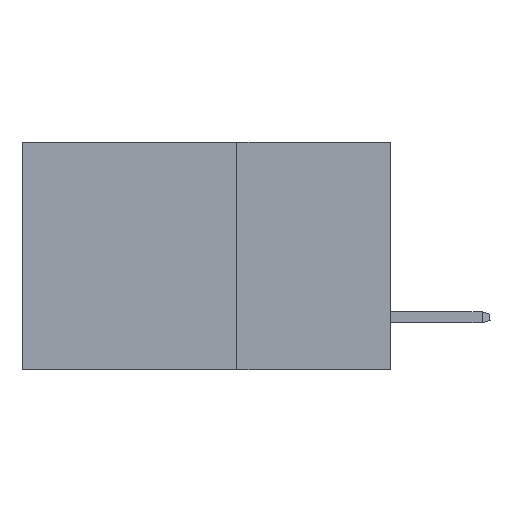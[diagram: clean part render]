
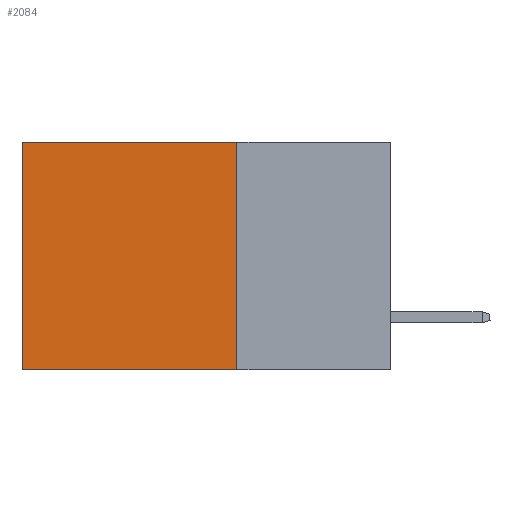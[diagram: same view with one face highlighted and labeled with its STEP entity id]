
A CAD part, left-side view. The second image highlights one B-rep face of the part: STEP entity #2084.
In plain terms, the highlighted planar face has unit normal (-1, 0, 0).
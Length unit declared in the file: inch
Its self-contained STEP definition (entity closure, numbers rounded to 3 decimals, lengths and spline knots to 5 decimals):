
#507 = DIRECTION ( 'NONE',  ( 0., 0., -1. ) ) ;
#755 = LINE ( 'NONE', #18049, #10126 ) ;
#2084 = ADVANCED_FACE ( 'NONE', ( #13882 ), #7536, .F. ) ;
#2392 = CARTESIAN_POINT ( 'NONE',  ( 0.2875, 0.25, -0.37 ) ) ;
#2902 = CARTESIAN_POINT ( 'NONE',  ( 0.2875, 0.25, 0. ) ) ;
#3713 = AXIS2_PLACEMENT_3D ( 'NONE', #2902, #4607, #16982 ) ;
#4004 = CARTESIAN_POINT ( 'NONE',  ( 0.2875, 0.6, 0. ) ) ;
#4607 = DIRECTION ( 'NONE',  ( 1., 0., 0. ) ) ;
#4824 = ORIENTED_EDGE ( 'NONE', *, *, #5139, .T. ) ;
#4842 = CARTESIAN_POINT ( 'NONE',  ( 0.2875, 0.25, 0. ) ) ;
#5139 = EDGE_CURVE ( 'NONE', #6283, #19271, #8482, .T. ) ;
#5158 = DIRECTION ( 'NONE',  ( 0., 0., -1. ) ) ;
#5989 = VECTOR ( 'NONE', #507, 39.37008 ) ;
#6265 = ORIENTED_EDGE ( 'NONE', *, *, #11631, .T. ) ;
#6283 = VERTEX_POINT ( 'NONE', #17704 ) ;
#6321 = VECTOR ( 'NONE', #9628, 39.37008 ) ;
#6827 = ORIENTED_EDGE ( 'NONE', *, *, #9391, .F. ) ;
#7020 = VERTEX_POINT ( 'NONE', #19019 ) ;
#7536 = PLANE ( 'NONE',  #3713 ) ;
#8482 = LINE ( 'NONE', #4842, #6321 ) ;
#9102 = VERTEX_POINT ( 'NONE', #2392 ) ;
#9391 = EDGE_CURVE ( 'NONE', #9102, #7020, #755, .T. ) ;
#9628 = DIRECTION ( 'NONE',  ( 0., 1., 0. ) ) ;
#10056 = LINE ( 'NONE', #15642, #5989 ) ;
#10126 = VECTOR ( 'NONE', #12023, 39.37008 ) ;
#11599 = EDGE_CURVE ( 'NONE', #6283, #9102, #10056, .T. ) ;
#11631 = EDGE_CURVE ( 'NONE', #19271, #7020, #13444, .T. ) ;
#11697 = ORIENTED_EDGE ( 'NONE', *, *, #11599, .F. ) ;
#12023 = DIRECTION ( 'NONE',  ( 0., 1., 0. ) ) ;
#13444 = LINE ( 'NONE', #14352, #13914 ) ;
#13882 = FACE_OUTER_BOUND ( 'NONE', #14234, .T. ) ;
#13914 = VECTOR ( 'NONE', #5158, 39.37008 ) ;
#14234 = EDGE_LOOP ( 'NONE', ( #6265, #6827, #11697, #4824 ) ) ;
#14352 = CARTESIAN_POINT ( 'NONE',  ( 0.2875, 0.6, 0. ) ) ;
#15642 = CARTESIAN_POINT ( 'NONE',  ( 0.2875, 0.25, 0. ) ) ;
#16982 = DIRECTION ( 'NONE',  ( 0., 0., -1. ) ) ;
#17704 = CARTESIAN_POINT ( 'NONE',  ( 0.2875, 0.25, 0. ) ) ;
#18049 = CARTESIAN_POINT ( 'NONE',  ( 0.2875, 0.25, -0.37 ) ) ;
#19019 = CARTESIAN_POINT ( 'NONE',  ( 0.2875, 0.6, -0.37 ) ) ;
#19271 = VERTEX_POINT ( 'NONE', #4004 ) ;
